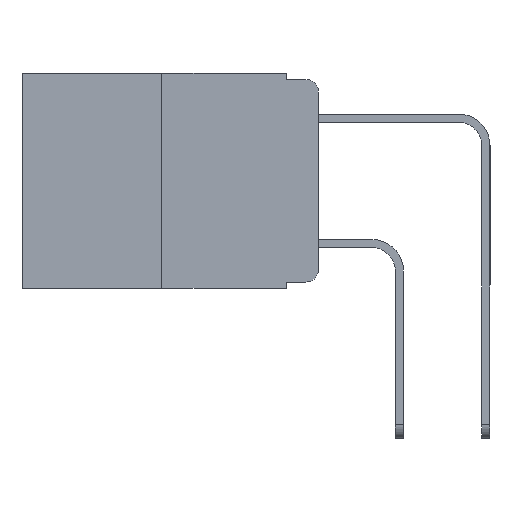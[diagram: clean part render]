
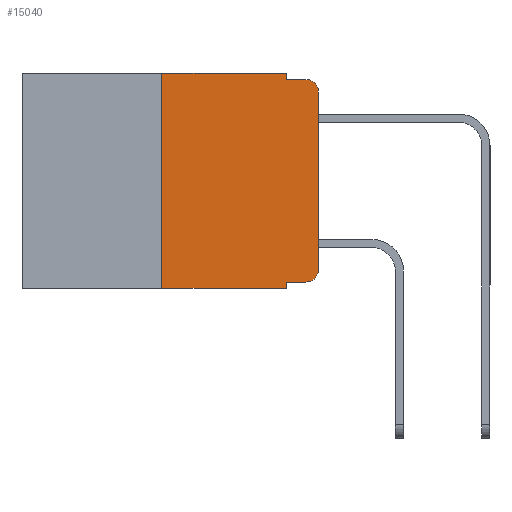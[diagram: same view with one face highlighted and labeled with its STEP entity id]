
A CAD part, left-side view. The second image highlights one B-rep face of the part: STEP entity #15040.
In plain terms, the highlighted planar face has unit normal (-1, 0, 0).
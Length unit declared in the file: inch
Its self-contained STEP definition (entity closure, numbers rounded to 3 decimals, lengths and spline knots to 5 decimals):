
#329 = VERTEX_POINT ( 'NONE', #7866 ) ;
#638 = DIRECTION ( 'NONE',  ( 1., 0., 0. ) ) ;
#896 = CARTESIAN_POINT ( 'NONE',  ( 0., 0.02, -0.333 ) ) ;
#1111 = EDGE_CURVE ( 'NONE', #15567, #13850, #17184, .T. ) ;
#1338 = VERTEX_POINT ( 'NONE', #13058 ) ;
#1348 = VERTEX_POINT ( 'NONE', #15416 ) ;
#1402 = ORIENTED_EDGE ( 'NONE', *, *, #10597, .F. ) ;
#1509 = ORIENTED_EDGE ( 'NONE', *, *, #7980, .T. ) ;
#1769 = VECTOR ( 'NONE', #15623, 39.37008 ) ;
#1971 = ORIENTED_EDGE ( 'NONE', *, *, #8747, .T. ) ;
#2167 = FACE_OUTER_BOUND ( 'NONE', #3225, .T. ) ;
#2419 = AXIS2_PLACEMENT_3D ( 'NONE', #7906, #16941, #9214 ) ;
#2435 = CARTESIAN_POINT ( 'NONE',  ( 0., 0.051, -0.01 ) ) ;
#2527 = LINE ( 'NONE', #14317, #5832 ) ;
#3010 = CIRCLE ( 'NONE', #12141, 0.02 ) ;
#3113 = ORIENTED_EDGE ( 'NONE', *, *, #6203, .T. ) ;
#3225 = EDGE_LOOP ( 'NONE', ( #4338, #10614, #10425, #10747, #3449, #10774, #1971, #1402, #1509, #3113 ) ) ;
#3289 = CARTESIAN_POINT ( 'NONE',  ( 0., 0.473, 0. ) ) ;
#3449 = ORIENTED_EDGE ( 'NONE', *, *, #15584, .F. ) ;
#3558 = VECTOR ( 'NONE', #11881, 39.37008 ) ;
#3696 = DIRECTION ( 'NONE',  ( -1., 0., 0. ) ) ;
#3730 = CARTESIAN_POINT ( 'NONE',  ( 0., 0.25, 0. ) ) ;
#3829 = CARTESIAN_POINT ( 'NONE',  ( 0., 0., 0. ) ) ;
#3835 = LINE ( 'NONE', #14135, #7493 ) ;
#4338 = ORIENTED_EDGE ( 'NONE', *, *, #1111, .T. ) ;
#5832 = VECTOR ( 'NONE', #9092, 39.37008 ) ;
#6020 = VECTOR ( 'NONE', #12058, 39.37008 ) ;
#6203 = EDGE_CURVE ( 'NONE', #7370, #15567, #3010, .T. ) ;
#6302 = DIRECTION ( 'NONE',  ( 0., -1., 0. ) ) ;
#6387 = CARTESIAN_POINT ( 'NONE',  ( 0., 0.25, 0. ) ) ;
#6519 = DIRECTION ( 'NONE',  ( 0., 0., 1. ) ) ;
#6925 = VERTEX_POINT ( 'NONE', #7927 ) ;
#7221 = CARTESIAN_POINT ( 'NONE',  ( 0., 0.051, -0.343 ) ) ;
#7370 = VERTEX_POINT ( 'NONE', #896 ) ;
#7460 = DIRECTION ( 'NONE',  ( 0., -1., 0. ) ) ;
#7493 = VECTOR ( 'NONE', #6302, 39.37008 ) ;
#7623 = VECTOR ( 'NONE', #7460, 39.37008 ) ;
#7697 = CARTESIAN_POINT ( 'NONE',  ( 0., 0.051, 0. ) ) ;
#7846 = AXIS2_PLACEMENT_3D ( 'NONE', #8930, #638, #10249 ) ;
#7866 = CARTESIAN_POINT ( 'NONE',  ( 0., 0.051, 0. ) ) ;
#7906 = CARTESIAN_POINT ( 'NONE',  ( 0., 0.02, -0.03 ) ) ;
#7927 = CARTESIAN_POINT ( 'NONE',  ( 0., 0.02, -0.01 ) ) ;
#7946 = VERTEX_POINT ( 'NONE', #14206 ) ;
#7980 = EDGE_CURVE ( 'NONE', #7946, #7370, #2527, .T. ) ;
#8182 = VECTOR ( 'NONE', #12947, 39.37008 ) ;
#8240 = CIRCLE ( 'NONE', #2419, 0.02 ) ;
#8747 = EDGE_CURVE ( 'NONE', #1338, #9699, #3835, .T. ) ;
#8930 = CARTESIAN_POINT ( 'NONE',  ( 0., 0.473, 0. ) ) ;
#9092 = DIRECTION ( 'NONE',  ( 0., -1., 0. ) ) ;
#9214 = DIRECTION ( 'NONE',  ( 0., 0., -1. ) ) ;
#9699 = VERTEX_POINT ( 'NONE', #7221 ) ;
#10025 = CARTESIAN_POINT ( 'NONE',  ( 0., 0., -0.313 ) ) ;
#10249 = DIRECTION ( 'NONE',  ( 0., 0., -1. ) ) ;
#10425 = ORIENTED_EDGE ( 'NONE', *, *, #14077, .F. ) ;
#10597 = EDGE_CURVE ( 'NONE', #7946, #9699, #12558, .T. ) ;
#10614 = ORIENTED_EDGE ( 'NONE', *, *, #15793, .T. ) ;
#10747 = ORIENTED_EDGE ( 'NONE', *, *, #13222, .F. ) ;
#10774 = ORIENTED_EDGE ( 'NONE', *, *, #11487, .F. ) ;
#11487 = EDGE_CURVE ( 'NONE', #1338, #13834, #15933, .T. ) ;
#11646 = LINE ( 'NONE', #7697, #8182 ) ;
#11724 = CARTESIAN_POINT ( 'NONE',  ( 0., 0.02, -0.313 ) ) ;
#11881 = DIRECTION ( 'NONE',  ( 0., -1., 0. ) ) ;
#12058 = DIRECTION ( 'NONE',  ( 0., 0., 1. ) ) ;
#12129 = VECTOR ( 'NONE', #6519, 39.37008 ) ;
#12141 = AXIS2_PLACEMENT_3D ( 'NONE', #11724, #3696, #13021 ) ;
#12558 = LINE ( 'NONE', #14366, #1769 ) ;
#12947 = DIRECTION ( 'NONE',  ( 0., 0., -1. ) ) ;
#13021 = DIRECTION ( 'NONE',  ( 0., 0., -1. ) ) ;
#13058 = CARTESIAN_POINT ( 'NONE',  ( 0., 0.25, -0.343 ) ) ;
#13222 = EDGE_CURVE ( 'NONE', #329, #1348, #11646, .T. ) ;
#13728 = LINE ( 'NONE', #3289, #7623 ) ;
#13834 = VERTEX_POINT ( 'NONE', #6387 ) ;
#13850 = VERTEX_POINT ( 'NONE', #15481 ) ;
#14077 = EDGE_CURVE ( 'NONE', #1348, #6925, #17144, .T. ) ;
#14135 = CARTESIAN_POINT ( 'NONE',  ( 0., 0.473, -0.343 ) ) ;
#14206 = CARTESIAN_POINT ( 'NONE',  ( 0., 0.051, -0.333 ) ) ;
#14317 = CARTESIAN_POINT ( 'NONE',  ( 0., 0.051, -0.333 ) ) ;
#14366 = CARTESIAN_POINT ( 'NONE',  ( 0., 0.051, 0. ) ) ;
#15040 = ADVANCED_FACE ( 'NONE', ( #2167 ), #16653, .F. ) ;
#15416 = CARTESIAN_POINT ( 'NONE',  ( 0., 0.051, -0.01 ) ) ;
#15481 = CARTESIAN_POINT ( 'NONE',  ( 0., 0., -0.03 ) ) ;
#15567 = VERTEX_POINT ( 'NONE', #10025 ) ;
#15584 = EDGE_CURVE ( 'NONE', #13834, #329, #13728, .T. ) ;
#15623 = DIRECTION ( 'NONE',  ( 0., 0., -1. ) ) ;
#15793 = EDGE_CURVE ( 'NONE', #13850, #6925, #8240, .T. ) ;
#15933 = LINE ( 'NONE', #3730, #12129 ) ;
#16653 = PLANE ( 'NONE',  #7846 ) ;
#16941 = DIRECTION ( 'NONE',  ( -1., 0., 0. ) ) ;
#17144 = LINE ( 'NONE', #2435, #3558 ) ;
#17184 = LINE ( 'NONE', #3829, #6020 ) ;
